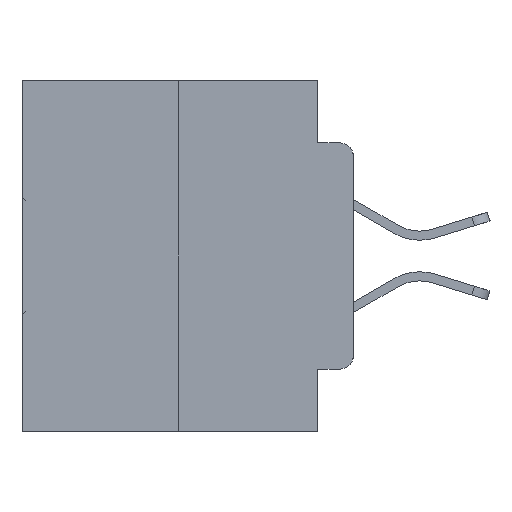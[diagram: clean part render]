
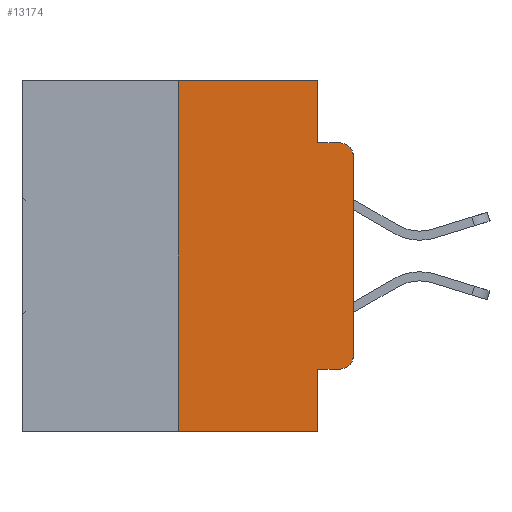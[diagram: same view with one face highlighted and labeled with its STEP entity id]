
A CAD part, left-side view. The second image highlights one B-rep face of the part: STEP entity #13174.
In plain terms, the highlighted planar face has unit normal (-1, 0, 0).
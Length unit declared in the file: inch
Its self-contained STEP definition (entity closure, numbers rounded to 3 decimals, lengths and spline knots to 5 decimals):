
#350 = DIRECTION ( 'NONE',  ( -1., 0., 0. ) ) ;
#439 = EDGE_CURVE ( 'NONE', #8599, #2762, #11289, .T. ) ;
#467 = VERTEX_POINT ( 'NONE', #8245 ) ;
#562 = CARTESIAN_POINT ( 'NONE',  ( 0., 0.051, -0.0885 ) ) ;
#818 = ORIENTED_EDGE ( 'NONE', *, *, #439, .T. ) ;
#2435 = ORIENTED_EDGE ( 'NONE', *, *, #25313, .T. ) ;
#2445 = VECTOR ( 'NONE', #19756, 39.37008 ) ;
#2762 = VERTEX_POINT ( 'NONE', #14783 ) ;
#3043 = DIRECTION ( 'NONE',  ( 0., -1., 0. ) ) ;
#3270 = VECTOR ( 'NONE', #12002, 39.37008 ) ;
#3671 = ORIENTED_EDGE ( 'NONE', *, *, #8849, .T. ) ;
#3990 = LINE ( 'NONE', #18551, #29159 ) ;
#4057 = ORIENTED_EDGE ( 'NONE', *, *, #26833, .F. ) ;
#4061 = PLANE ( 'NONE',  #17230 ) ;
#4069 = LINE ( 'NONE', #24260, #3270 ) ;
#5636 = LINE ( 'NONE', #12765, #11550 ) ;
#5744 = VERTEX_POINT ( 'NONE', #7646 ) ;
#6279 = CIRCLE ( 'NONE', #25913, 0.02 ) ;
#6520 = VERTEX_POINT ( 'NONE', #23572 ) ;
#6950 = CARTESIAN_POINT ( 'NONE',  ( 0., 0.051, -0.4115 ) ) ;
#7646 = CARTESIAN_POINT ( 'NONE',  ( 0., 0.051, 0. ) ) ;
#7907 = DIRECTION ( 'NONE',  ( 0., 0., 1. ) ) ;
#8245 = CARTESIAN_POINT ( 'NONE',  ( 0., 0.25, -0.5 ) ) ;
#8490 = LINE ( 'NONE', #22903, #14342 ) ;
#8599 = VERTEX_POINT ( 'NONE', #19602 ) ;
#8849 = EDGE_CURVE ( 'NONE', #6520, #8599, #6279, .T. ) ;
#8912 = EDGE_CURVE ( 'NONE', #11858, #29003, #30123, .T. ) ;
#9171 = DIRECTION ( 'NONE',  ( 0., 0., -1. ) ) ;
#10646 = FACE_OUTER_BOUND ( 'NONE', #12414, .T. ) ;
#10809 = CARTESIAN_POINT ( 'NONE',  ( 0., 0.02, -0.0885 ) ) ;
#11289 = LINE ( 'NONE', #30098, #17896 ) ;
#11436 = CARTESIAN_POINT ( 'NONE',  ( 0., 0.02, -0.1085 ) ) ;
#11518 = AXIS2_PLACEMENT_3D ( 'NONE', #11436, #28573, #13940 ) ;
#11532 = CARTESIAN_POINT ( 'NONE',  ( 0., 0.051, -0.5 ) ) ;
#11550 = VECTOR ( 'NONE', #12875, 39.37008 ) ;
#11591 = CARTESIAN_POINT ( 'NONE',  ( 0., 0.473, 0. ) ) ;
#11858 = VERTEX_POINT ( 'NONE', #14810 ) ;
#11875 = EDGE_CURVE ( 'NONE', #29270, #6520, #23917, .T. ) ;
#12002 = DIRECTION ( 'NONE',  ( 0., 0., -1. ) ) ;
#12414 = EDGE_LOOP ( 'NONE', ( #818, #2435, #15889, #23142, #4057, #23907, #18939, #31828, #22778, #3671 ) ) ;
#12765 = CARTESIAN_POINT ( 'NONE',  ( 0., 0.25, 0. ) ) ;
#12875 = DIRECTION ( 'NONE',  ( 0., 0., 1. ) ) ;
#13174 = ADVANCED_FACE ( 'NONE', ( #10646 ), #4061, .F. ) ;
#13940 = DIRECTION ( 'NONE',  ( 0., 0., -1. ) ) ;
#14342 = VECTOR ( 'NONE', #3043, 39.37008 ) ;
#14758 = CARTESIAN_POINT ( 'NONE',  ( 0., 0.25, 0. ) ) ;
#14783 = CARTESIAN_POINT ( 'NONE',  ( 0., 0., -0.1085 ) ) ;
#14810 = CARTESIAN_POINT ( 'NONE',  ( 0., 0.051, -0.0885 ) ) ;
#15517 = CARTESIAN_POINT ( 'NONE',  ( 0., 0.02, -0.3915 ) ) ;
#15889 = ORIENTED_EDGE ( 'NONE', *, *, #8912, .F. ) ;
#16011 = VERTEX_POINT ( 'NONE', #14758 ) ;
#16286 = EDGE_CURVE ( 'NONE', #467, #27926, #8490, .T. ) ;
#16643 = EDGE_CURVE ( 'NONE', #29270, #27926, #4069, .T. ) ;
#17230 = AXIS2_PLACEMENT_3D ( 'NONE', #21533, #23964, #9171 ) ;
#17247 = VECTOR ( 'NONE', #23111, 39.37008 ) ;
#17305 = CARTESIAN_POINT ( 'NONE',  ( 0., 0.051, -0.4115 ) ) ;
#17896 = VECTOR ( 'NONE', #7907, 39.37008 ) ;
#17980 = DIRECTION ( 'NONE',  ( 0., 0., -1. ) ) ;
#18551 = CARTESIAN_POINT ( 'NONE',  ( 0., 0.051, 0. ) ) ;
#18939 = ORIENTED_EDGE ( 'NONE', *, *, #16286, .T. ) ;
#19061 = DIRECTION ( 'NONE',  ( 0., -1., 0. ) ) ;
#19602 = CARTESIAN_POINT ( 'NONE',  ( 0., 0., -0.3915 ) ) ;
#19756 = DIRECTION ( 'NONE',  ( 0., -1., 0. ) ) ;
#20879 = EDGE_CURVE ( 'NONE', #467, #16011, #5636, .T. ) ;
#21029 = DIRECTION ( 'NONE',  ( 0., 0., -1. ) ) ;
#21533 = CARTESIAN_POINT ( 'NONE',  ( 0., 0.473, 0. ) ) ;
#21831 = LINE ( 'NONE', #11591, #28251 ) ;
#22778 = ORIENTED_EDGE ( 'NONE', *, *, #11875, .T. ) ;
#22903 = CARTESIAN_POINT ( 'NONE',  ( 0., 0.473, -0.5 ) ) ;
#23111 = DIRECTION ( 'NONE',  ( 0., -1., 0. ) ) ;
#23142 = ORIENTED_EDGE ( 'NONE', *, *, #30717, .F. ) ;
#23572 = CARTESIAN_POINT ( 'NONE',  ( 0., 0.02, -0.4115 ) ) ;
#23907 = ORIENTED_EDGE ( 'NONE', *, *, #20879, .F. ) ;
#23917 = LINE ( 'NONE', #17305, #2445 ) ;
#23964 = DIRECTION ( 'NONE',  ( 1., 0., 0. ) ) ;
#24260 = CARTESIAN_POINT ( 'NONE',  ( 0., 0.051, 0. ) ) ;
#25313 = EDGE_CURVE ( 'NONE', #2762, #29003, #25567, .T. ) ;
#25567 = CIRCLE ( 'NONE', #11518, 0.02 ) ;
#25913 = AXIS2_PLACEMENT_3D ( 'NONE', #15517, #350, #17980 ) ;
#26833 = EDGE_CURVE ( 'NONE', #16011, #5744, #21831, .T. ) ;
#27926 = VERTEX_POINT ( 'NONE', #11532 ) ;
#28251 = VECTOR ( 'NONE', #19061, 39.37008 ) ;
#28573 = DIRECTION ( 'NONE',  ( -1., 0., 0. ) ) ;
#29003 = VERTEX_POINT ( 'NONE', #10809 ) ;
#29159 = VECTOR ( 'NONE', #21029, 39.37008 ) ;
#29270 = VERTEX_POINT ( 'NONE', #6950 ) ;
#30098 = CARTESIAN_POINT ( 'NONE',  ( 0., 0., 0. ) ) ;
#30123 = LINE ( 'NONE', #562, #17247 ) ;
#30717 = EDGE_CURVE ( 'NONE', #5744, #11858, #3990, .T. ) ;
#31828 = ORIENTED_EDGE ( 'NONE', *, *, #16643, .F. ) ;
